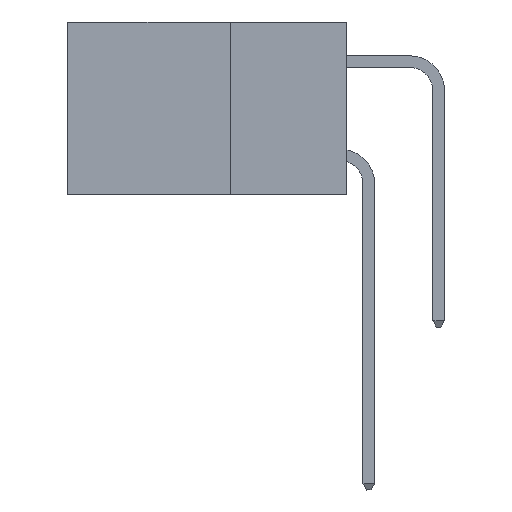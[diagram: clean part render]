
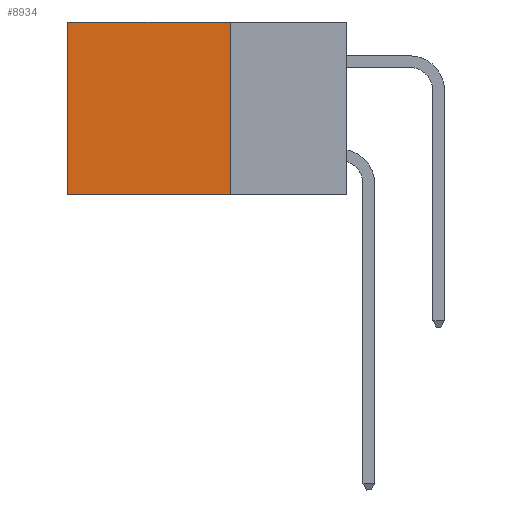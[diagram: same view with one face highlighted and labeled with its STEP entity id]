
A CAD part, left-side view. The second image highlights one B-rep face of the part: STEP entity #8934.
In plain terms, the highlighted planar face has unit normal (-1, 0, 0).
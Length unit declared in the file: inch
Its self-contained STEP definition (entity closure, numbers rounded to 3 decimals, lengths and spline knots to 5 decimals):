
#1086 = DIRECTION ( 'NONE',  ( 0., 0., -1. ) ) ;
#1293 = CARTESIAN_POINT ( 'NONE',  ( 0.2875, 0.25, 0. ) ) ;
#1364 = LINE ( 'NONE', #8064, #10099 ) ;
#1792 = DIRECTION ( 'NONE',  ( 0., 1., 0. ) ) ;
#1830 = CARTESIAN_POINT ( 'NONE',  ( 0.2875, 0.25, 0. ) ) ;
#1895 = VECTOR ( 'NONE', #8374, 39.37008 ) ;
#2079 = FACE_OUTER_BOUND ( 'NONE', #2178, .T. ) ;
#2178 = EDGE_LOOP ( 'NONE', ( #5023, #5448, #3407, #13686 ) ) ;
#3044 = VERTEX_POINT ( 'NONE', #7444 ) ;
#3407 = ORIENTED_EDGE ( 'NONE', *, *, #3922, .F. ) ;
#3554 = VERTEX_POINT ( 'NONE', #9248 ) ;
#3922 = EDGE_CURVE ( 'NONE', #8762, #10756, #1364, .T. ) ;
#4279 = EDGE_CURVE ( 'NONE', #3554, #3044, #12096, .T. ) ;
#5023 = ORIENTED_EDGE ( 'NONE', *, *, #4279, .T. ) ;
#5404 = CARTESIAN_POINT ( 'NONE',  ( 0.2875, 0.25, 0. ) ) ;
#5448 = ORIENTED_EDGE ( 'NONE', *, *, #11761, .F. ) ;
#6043 = CARTESIAN_POINT ( 'NONE',  ( 0.2875, 0.6, 0. ) ) ;
#6159 = CARTESIAN_POINT ( 'NONE',  ( 0.2875, 0.25, -0.37 ) ) ;
#6516 = EDGE_CURVE ( 'NONE', #8762, #3554, #7866, .T. ) ;
#6763 = VECTOR ( 'NONE', #9406, 39.37008 ) ;
#7408 = AXIS2_PLACEMENT_3D ( 'NONE', #5404, #12338, #14681 ) ;
#7444 = CARTESIAN_POINT ( 'NONE',  ( 0.2875, 0.6, -0.37 ) ) ;
#7866 = LINE ( 'NONE', #1293, #6763 ) ;
#8064 = CARTESIAN_POINT ( 'NONE',  ( 0.2875, 0.25, 0. ) ) ;
#8374 = DIRECTION ( 'NONE',  ( 0., 0., -1. ) ) ;
#8762 = VERTEX_POINT ( 'NONE', #1830 ) ;
#8934 = ADVANCED_FACE ( 'NONE', ( #2079 ), #11294, .F. ) ;
#9248 = CARTESIAN_POINT ( 'NONE',  ( 0.2875, 0.6, 0. ) ) ;
#9406 = DIRECTION ( 'NONE',  ( 0., 1., 0. ) ) ;
#10099 = VECTOR ( 'NONE', #1086, 39.37008 ) ;
#10756 = VERTEX_POINT ( 'NONE', #12242 ) ;
#11294 = PLANE ( 'NONE',  #7408 ) ;
#11761 = EDGE_CURVE ( 'NONE', #10756, #3044, #12522, .T. ) ;
#12096 = LINE ( 'NONE', #6043, #1895 ) ;
#12242 = CARTESIAN_POINT ( 'NONE',  ( 0.2875, 0.25, -0.37 ) ) ;
#12338 = DIRECTION ( 'NONE',  ( 1., 0., 0. ) ) ;
#12522 = LINE ( 'NONE', #6159, #13995 ) ;
#13686 = ORIENTED_EDGE ( 'NONE', *, *, #6516, .T. ) ;
#13995 = VECTOR ( 'NONE', #1792, 39.37008 ) ;
#14681 = DIRECTION ( 'NONE',  ( 0., 0., -1. ) ) ;
